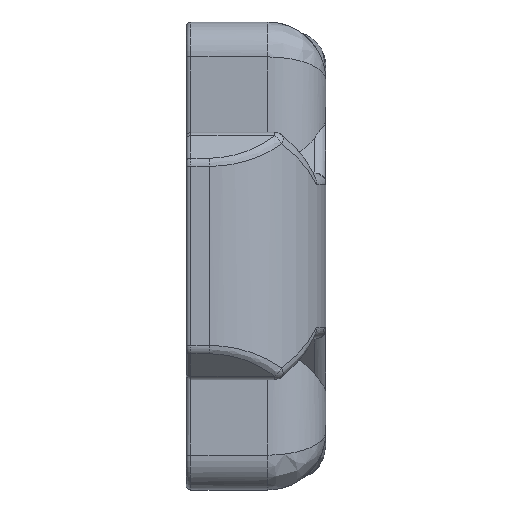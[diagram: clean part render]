
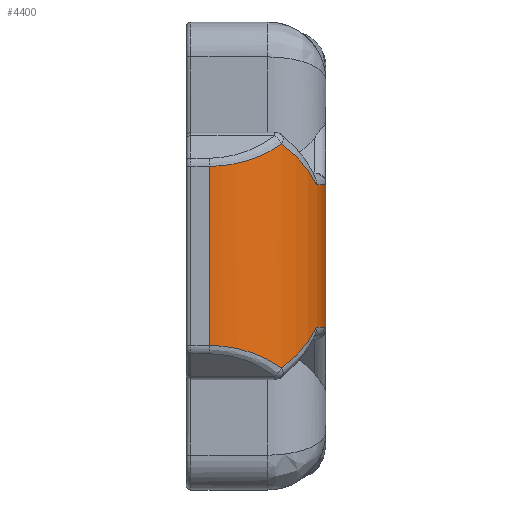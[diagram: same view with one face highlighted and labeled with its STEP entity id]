
A CAD part, front view. The second image highlights one B-rep face of the part: STEP entity #4400.
In plain terms, the highlighted cylindrical face has radius 10 mm (diameter 20 mm), a partial arc.
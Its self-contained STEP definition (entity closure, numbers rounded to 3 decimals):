
#17 = CIRCLE ( 'NONE', #2198, 10. ) ;
#19 = CARTESIAN_POINT ( 'NONE',  ( 115.827, -7.031, 8.7 ) ) ;
#225 = CARTESIAN_POINT ( 'NONE',  ( 112.771, -9.447, 8.388 ) ) ;
#234 = CARTESIAN_POINT ( 'NONE',  ( 118.318, -0.22, 6.422 ) ) ;
#294 = DIRECTION ( 'NONE',  ( 0., 0., -1. ) ) ;
#471 = CARTESIAN_POINT ( 'NONE',  ( 118.318, -0.333, -6.313 ) ) ;
#521 = CARTESIAN_POINT ( 'NONE',  ( 118.318, -0.22, -6.415 ) ) ;
#657 = EDGE_CURVE ( 'NONE', #2272, #935, #2679, .T. ) ;
#702 = EDGE_CURVE ( 'NONE', #3686, #2876, #1891, .T. ) ;
#748 =( BOUNDED_CURVE ( )  B_SPLINE_CURVE ( 3, ( #2292, #471, #3263, #3793 ),
 .UNSPECIFIED., .F., .T. ) 
 B_SPLINE_CURVE_WITH_KNOTS ( ( 4, 4 ),
 ( 1.571, 1.605 ),
 .UNSPECIFIED. ) 
 CURVE ( )  GEOMETRIC_REPRESENTATION_ITEM ( )  RATIONAL_B_SPLINE_CURVE ( ( 1., 1., 1., 1. ) ) 
 REPRESENTATION_ITEM ( '' )  );
#935 = VERTEX_POINT ( 'NONE', #1192 ) ;
#1067 = DIRECTION ( 'NONE',  ( 0.981, -0.193, 0. ) ) ;
#1134 = CARTESIAN_POINT ( 'NONE',  ( 114.52, -8.064, -9.614 ) ) ;
#1150 = DIRECTION ( 'NONE',  ( 0.707, -0.707, 0. ) ) ;
#1192 = CARTESIAN_POINT ( 'NONE',  ( 117.521, -4.133, -6.109 ) ) ;
#1341 = EDGE_CURVE ( 'NONE', #3965, #2272, #748, .T. ) ;
#1388 = EDGE_CURVE ( 'NONE', #2876, #2674, #3273, .T. ) ;
#1514 = DIRECTION ( 'NONE',  ( 0.981, -0.193, 0. ) ) ;
#1534 = ORIENTED_EDGE ( 'NONE', *, *, #4024, .T. ) ;
#1593 = DIRECTION ( 'NONE',  ( 0., 0., 1. ) ) ;
#1609 = CARTESIAN_POINT ( 'NONE',  ( 114.52, -8.064, -9.614 ) ) ;
#1687 =( BOUNDED_CURVE ( )  B_SPLINE_CURVE ( 3, ( #2523, #4990, #5938, #3494 ),
 .UNSPECIFIED., .F., .T. ) 
 B_SPLINE_CURVE_WITH_KNOTS ( ( 4, 4 ),
 ( 4.678, 4.712 ),
 .UNSPECIFIED. ) 
 CURVE ( )  GEOMETRIC_REPRESENTATION_ITEM ( )  RATIONAL_B_SPLINE_CURVE ( ( 1., 1., 1., 1. ) ) 
 REPRESENTATION_ITEM ( '' )  );
#1891 = B_SPLINE_CURVE_WITH_KNOTS ( 'NONE', 3,
 ( #4333, #4965, #225, #3560 ),
 .UNSPECIFIED., .F., .F.,
 ( 4, 4 ),
 ( 0., 1. ),
 .UNSPECIFIED. ) ;
#1903 = CARTESIAN_POINT ( 'NONE',  ( 117.521, -4.133, 6.116 ) ) ;
#2052 = VERTEX_POINT ( 'NONE', #4948 ) ;
#2141 = ORIENTED_EDGE ( 'NONE', *, *, #2737, .F. ) ;
#2198 = AXIS2_PLACEMENT_3D ( 'NONE', #3381, #4854, #1067 ) ;
#2272 = VERTEX_POINT ( 'NONE', #5584 ) ;
#2292 = CARTESIAN_POINT ( 'NONE',  ( 118.318, -0.22, -6.415 ) ) ;
#2426 = CARTESIAN_POINT ( 'NONE',  ( 108.318, -10.22, 7.699 ) ) ;
#2523 = CARTESIAN_POINT ( 'NONE',  ( 118.312, -0.56, 6.116 ) ) ;
#2570 = CARTESIAN_POINT ( 'NONE',  ( 116.869, -5.666, -7.476 ) ) ;
#2593 = CARTESIAN_POINT ( 'NONE',  ( 117.521, -4.133, -6.109 ) ) ;
#2664 = CARTESIAN_POINT ( 'NONE',  ( 108.318, -10.22, -7.692 ) ) ;
#2674 = VERTEX_POINT ( 'NONE', #2686 ) ;
#2679 = CIRCLE ( 'NONE', #3658, 10. ) ;
#2686 = CARTESIAN_POINT ( 'NONE',  ( 117.521, -4.133, 6.116 ) ) ;
#2705 = FACE_OUTER_BOUND ( 'NONE', #4830, .T. ) ;
#2714 = B_SPLINE_CURVE_WITH_KNOTS ( 'NONE', 3,
 ( #1134, #5901, #4052, #3033 ),
 .UNSPECIFIED., .F., .F.,
 ( 4, 4 ),
 ( 0., 1. ),
 .UNSPECIFIED. ) ;
#2737 = EDGE_CURVE ( 'NONE', #2052, #4145, #1687, .T. ) ;
#2743 = CARTESIAN_POINT ( 'NONE',  ( 108.318, -10.22, 1.365 ) ) ;
#2795 = ORIENTED_EDGE ( 'NONE', *, *, #5132, .T. ) ;
#2876 = VERTEX_POINT ( 'NONE', #4607 ) ;
#2916 = LINE ( 'NONE', #2743, #4582 ) ;
#2933 = DIRECTION ( 'NONE',  ( 0., 0., -1. ) ) ;
#3033 = CARTESIAN_POINT ( 'NONE',  ( 108.318, -10.22, -7.692 ) ) ;
#3036 = VERTEX_POINT ( 'NONE', #5116 ) ;
#3094 = ORIENTED_EDGE ( 'NONE', *, *, #4060, .F. ) ;
#3118 = CARTESIAN_POINT ( 'NONE',  ( 108.318, -0.22, 1.365 ) ) ;
#3185 = ORIENTED_EDGE ( 'NONE', *, *, #657, .F. ) ;
#3263 = CARTESIAN_POINT ( 'NONE',  ( 118.316, -0.447, -6.211 ) ) ;
#3273 = B_SPLINE_CURVE_WITH_KNOTS ( 'NONE', 3,
 ( #3838, #19, #5734, #1903 ),
 .UNSPECIFIED., .F., .F.,
 ( 4, 4 ),
 ( 0., 1. ),
 .UNSPECIFIED. ) ;
#3367 = CARTESIAN_POINT ( 'NONE',  ( 108.318, -0.22, -6.109 ) ) ;
#3381 = CARTESIAN_POINT ( 'NONE',  ( 108.318, -0.22, 6.116 ) ) ;
#3402 = VERTEX_POINT ( 'NONE', #2664 ) ;
#3494 = CARTESIAN_POINT ( 'NONE',  ( 118.318, -0.22, 6.422 ) ) ;
#3534 = ORIENTED_EDGE ( 'NONE', *, *, #1388, .F. ) ;
#3560 = CARTESIAN_POINT ( 'NONE',  ( 114.52, -8.064, 9.621 ) ) ;
#3658 = AXIS2_PLACEMENT_3D ( 'NONE', #3367, #2933, #1514 ) ;
#3682 = AXIS2_PLACEMENT_3D ( 'NONE', #3118, #5426, #1150 ) ;
#3686 = VERTEX_POINT ( 'NONE', #2426 ) ;
#3793 = CARTESIAN_POINT ( 'NONE',  ( 118.312, -0.56, -6.109 ) ) ;
#3802 = EDGE_CURVE ( 'NONE', #935, #3036, #5368, .T. ) ;
#3838 = CARTESIAN_POINT ( 'NONE',  ( 114.52, -8.064, 9.621 ) ) ;
#3880 = EDGE_CURVE ( 'NONE', #2674, #2052, #17, .T. ) ;
#3965 = VERTEX_POINT ( 'NONE', #521 ) ;
#4024 = EDGE_CURVE ( 'NONE', #3965, #4145, #5906, .T. ) ;
#4052 = CARTESIAN_POINT ( 'NONE',  ( 110.548, -10.22, -7.692 ) ) ;
#4060 = EDGE_CURVE ( 'NONE', #3036, #3402, #2714, .T. ) ;
#4145 = VERTEX_POINT ( 'NONE', #234 ) ;
#4169 = ORIENTED_EDGE ( 'NONE', *, *, #3880, .F. ) ;
#4182 = ORIENTED_EDGE ( 'NONE', *, *, #702, .F. ) ;
#4333 = CARTESIAN_POINT ( 'NONE',  ( 108.318, -10.22, 7.699 ) ) ;
#4400 = ADVANCED_FACE ( 'NONE', ( #2705 ), #6134, .T. ) ;
#4440 = ORIENTED_EDGE ( 'NONE', *, *, #3802, .F. ) ;
#4582 = VECTOR ( 'NONE', #294, 1000. ) ;
#4607 = CARTESIAN_POINT ( 'NONE',  ( 114.52, -8.064, 9.621 ) ) ;
#4830 = EDGE_LOOP ( 'NONE', ( #3094, #4440, #3185, #6023, #1534, #2141, #4169, #3534, #4182, #2795 ) ) ;
#4854 = DIRECTION ( 'NONE',  ( 0., 0., 1. ) ) ;
#4942 = CARTESIAN_POINT ( 'NONE',  ( 115.827, -7.031, -8.693 ) ) ;
#4948 = CARTESIAN_POINT ( 'NONE',  ( 118.312, -0.56, 6.116 ) ) ;
#4965 = CARTESIAN_POINT ( 'NONE',  ( 110.548, -10.22, 7.699 ) ) ;
#4990 = CARTESIAN_POINT ( 'NONE',  ( 118.316, -0.447, 6.218 ) ) ;
#5116 = CARTESIAN_POINT ( 'NONE',  ( 114.52, -8.064, -9.614 ) ) ;
#5132 = EDGE_CURVE ( 'NONE', #3686, #3402, #2916, .T. ) ;
#5368 = B_SPLINE_CURVE_WITH_KNOTS ( 'NONE', 3,
 ( #2593, #2570, #4942, #1609 ),
 .UNSPECIFIED., .F., .F.,
 ( 4, 4 ),
 ( 0., 1. ),
 .UNSPECIFIED. ) ;
#5407 = CARTESIAN_POINT ( 'NONE',  ( 118.318, -0.22, 1.365 ) ) ;
#5426 = DIRECTION ( 'NONE',  ( 0., 0., 1. ) ) ;
#5584 = CARTESIAN_POINT ( 'NONE',  ( 118.312, -0.56, -6.109 ) ) ;
#5602 = VECTOR ( 'NONE', #1593, 1000. ) ;
#5734 = CARTESIAN_POINT ( 'NONE',  ( 116.869, -5.666, 7.483 ) ) ;
#5901 = CARTESIAN_POINT ( 'NONE',  ( 112.771, -9.447, -8.381 ) ) ;
#5906 = LINE ( 'NONE', #5407, #5602 ) ;
#5938 = CARTESIAN_POINT ( 'NONE',  ( 118.318, -0.333, 6.32 ) ) ;
#6023 = ORIENTED_EDGE ( 'NONE', *, *, #1341, .F. ) ;
#6134 = CYLINDRICAL_SURFACE ( 'NONE', #3682, 10. ) ;
